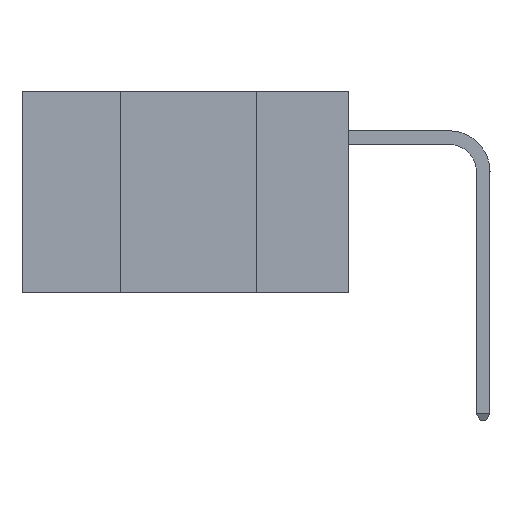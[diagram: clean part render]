
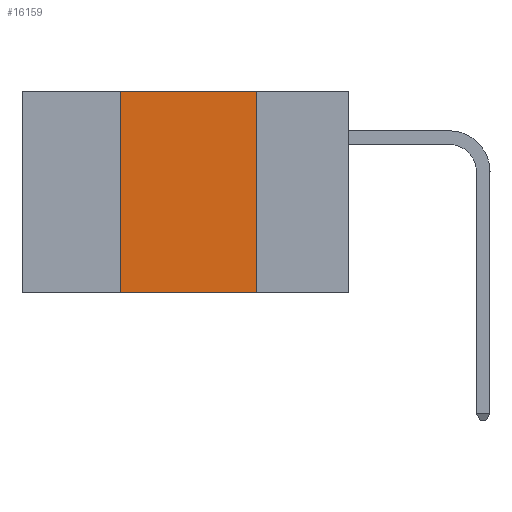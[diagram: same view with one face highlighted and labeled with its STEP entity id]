
A CAD part, left-side view. The second image highlights one B-rep face of the part: STEP entity #16159.
In plain terms, the highlighted planar face has unit normal (-1, 0, 0).
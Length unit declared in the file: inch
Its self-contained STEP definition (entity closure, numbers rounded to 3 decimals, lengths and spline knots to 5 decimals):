
#104 = AXIS2_PLACEMENT_3D ( 'NONE', #6563, #16021, #7985 ) ;
#1229 = VERTEX_POINT ( 'NONE', #6741 ) ;
#1428 = LINE ( 'NONE', #9755, #4649 ) ;
#2554 = VERTEX_POINT ( 'NONE', #14401 ) ;
#3094 = VERTEX_POINT ( 'NONE', #17017 ) ;
#3742 = VECTOR ( 'NONE', #5402, 39.37008 ) ;
#4037 = CARTESIAN_POINT ( 'NONE',  ( 0., 0.17, 0. ) ) ;
#4649 = VECTOR ( 'NONE', #16542, 39.37008 ) ;
#4793 = EDGE_CURVE ( 'NONE', #3094, #2554, #5866, .T. ) ;
#5402 = DIRECTION ( 'NONE',  ( 0., 0., -1. ) ) ;
#5866 = LINE ( 'NONE', #17543, #9101 ) ;
#6315 = EDGE_CURVE ( 'NONE', #1229, #7045, #15401, .T. ) ;
#6563 = CARTESIAN_POINT ( 'NONE',  ( 0., 0.6, 0. ) ) ;
#6741 = CARTESIAN_POINT ( 'NONE',  ( 0., 0.42, 0. ) ) ;
#7045 = VERTEX_POINT ( 'NONE', #8797 ) ;
#7650 = ORIENTED_EDGE ( 'NONE', *, *, #10649, .F. ) ;
#7985 = DIRECTION ( 'NONE',  ( 0., 0., -1. ) ) ;
#8262 = VECTOR ( 'NONE', #10367, 39.37008 ) ;
#8649 = CARTESIAN_POINT ( 'NONE',  ( 0., 0.6, 0. ) ) ;
#8797 = CARTESIAN_POINT ( 'NONE',  ( 0., 0.17, 0. ) ) ;
#9101 = VECTOR ( 'NONE', #16785, 39.37008 ) ;
#9755 = CARTESIAN_POINT ( 'NONE',  ( 0., 0.42, 0. ) ) ;
#10367 = DIRECTION ( 'NONE',  ( 0., -1., 0. ) ) ;
#10649 = EDGE_CURVE ( 'NONE', #3094, #1229, #1428, .T. ) ;
#11836 = ORIENTED_EDGE ( 'NONE', *, *, #4793, .T. ) ;
#12370 = EDGE_CURVE ( 'NONE', #7045, #2554, #14592, .T. ) ;
#13277 = ORIENTED_EDGE ( 'NONE', *, *, #6315, .F. ) ;
#14401 = CARTESIAN_POINT ( 'NONE',  ( 0., 0.17, -0.37 ) ) ;
#14518 = EDGE_LOOP ( 'NONE', ( #17256, #13277, #7650, #11836 ) ) ;
#14592 = LINE ( 'NONE', #4037, #3742 ) ;
#14678 = PLANE ( 'NONE',  #104 ) ;
#14679 = FACE_OUTER_BOUND ( 'NONE', #14518, .T. ) ;
#15401 = LINE ( 'NONE', #8649, #8262 ) ;
#16021 = DIRECTION ( 'NONE',  ( 1., 0., 0. ) ) ;
#16159 = ADVANCED_FACE ( 'NONE', ( #14679 ), #14678, .F. ) ;
#16542 = DIRECTION ( 'NONE',  ( 0., 0., 1. ) ) ;
#16785 = DIRECTION ( 'NONE',  ( 0., -1., 0. ) ) ;
#17017 = CARTESIAN_POINT ( 'NONE',  ( 0., 0.42, -0.37 ) ) ;
#17256 = ORIENTED_EDGE ( 'NONE', *, *, #12370, .F. ) ;
#17543 = CARTESIAN_POINT ( 'NONE',  ( 0., 0.6, -0.37 ) ) ;
